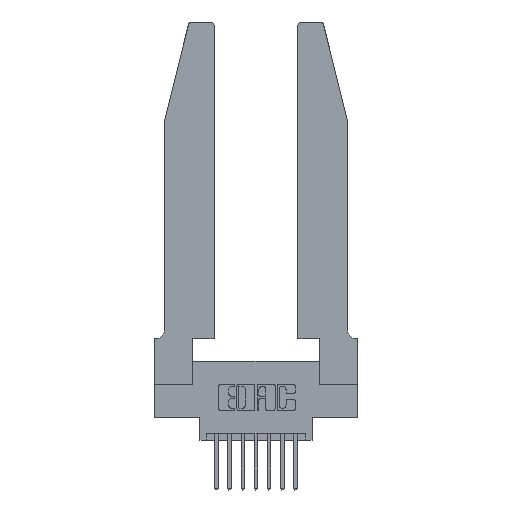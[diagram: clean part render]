
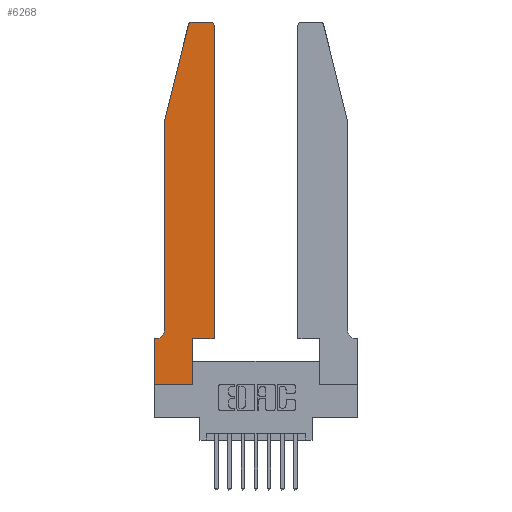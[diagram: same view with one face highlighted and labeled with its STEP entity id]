
A CAD part, top view. The second image highlights one B-rep face of the part: STEP entity #6268.
In plain terms, the highlighted planar face has unit normal (0, 0, 1).
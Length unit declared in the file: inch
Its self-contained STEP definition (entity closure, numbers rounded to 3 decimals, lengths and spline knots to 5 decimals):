
#168 = PLANE ( 'NONE',  #6182 ) ;
#201 = LINE ( 'NONE', #10219, #4741 ) ;
#325 = CARTESIAN_POINT ( 'NONE',  ( 0.2605, 2.75, 0.37 ) ) ;
#333 = CARTESIAN_POINT ( 'NONE',  ( 0.25487, 2.72718, 0.37 ) ) ;
#582 = EDGE_CURVE ( 'NONE', #6968, #1388, #7446, .T. ) ;
#644 = AXIS2_PLACEMENT_3D ( 'NONE', #13513, #14872, #884 ) ;
#813 = AXIS2_PLACEMENT_3D ( 'NONE', #11903, #7226, #1496 ) ;
#844 = ORIENTED_EDGE ( 'NONE', *, *, #5226, .T. ) ;
#884 = DIRECTION ( 'NONE',  ( 1., 0., 0. ) ) ;
#895 = LINE ( 'NONE', #1168, #10891 ) ;
#1052 = CIRCLE ( 'NONE', #7190, 0.03 ) ;
#1168 = CARTESIAN_POINT ( 'NONE',  ( 0.0755, 0.35, 0.37 ) ) ;
#1303 = ORIENTED_EDGE ( 'NONE', *, *, #3706, .T. ) ;
#1388 = VERTEX_POINT ( 'NONE', #13050 ) ;
#1453 = LINE ( 'NONE', #325, #6697 ) ;
#1496 = DIRECTION ( 'NONE',  ( -1., 0., 0. ) ) ;
#1751 = ORIENTED_EDGE ( 'NONE', *, *, #6201, .T. ) ;
#1813 = CARTESIAN_POINT ( 'NONE',  ( 0.2865, 0.35, 0.37 ) ) ;
#1966 = VECTOR ( 'NONE', #7671, 39.37008 ) ;
#2063 = EDGE_CURVE ( 'NONE', #12462, #11241, #1453, .T. ) ;
#2117 = ORIENTED_EDGE ( 'NONE', *, *, #2491, .T. ) ;
#2491 = EDGE_CURVE ( 'NONE', #1388, #6973, #895, .T. ) ;
#2629 = DIRECTION ( 'NONE',  ( 0., -1., 0. ) ) ;
#2671 = LINE ( 'NONE', #13246, #11955 ) ;
#2786 = CARTESIAN_POINT ( 'NONE',  ( 0., 0., 0.37 ) ) ;
#2813 = DIRECTION ( 'NONE',  ( 1., 0., 0. ) ) ;
#2815 = CARTESIAN_POINT ( 'NONE',  ( 0., 0., 0.37 ) ) ;
#3256 = CARTESIAN_POINT ( 'NONE',  ( 0.2865, 0., 0.37 ) ) ;
#3304 = DIRECTION ( 'NONE',  ( 0., 1., 0. ) ) ;
#3486 = CARTESIAN_POINT ( 'NONE',  ( 0.0755, 2., 0.37 ) ) ;
#3706 = EDGE_CURVE ( 'NONE', #4061, #13026, #6099, .T. ) ;
#3742 = LINE ( 'NONE', #2786, #11026 ) ;
#3994 = DIRECTION ( 'NONE',  ( -1., 0., 0. ) ) ;
#4061 = VERTEX_POINT ( 'NONE', #3256 ) ;
#4136 = DIRECTION ( 'NONE',  ( 0., 1., 0. ) ) ;
#4289 = EDGE_CURVE ( 'NONE', #11241, #5886, #12460, .T. ) ;
#4650 = DIRECTION ( 'NONE',  ( 1., 0., 0. ) ) ;
#4741 = VECTOR ( 'NONE', #3304, 39.37008 ) ;
#4876 = VECTOR ( 'NONE', #2813, 39.37008 ) ;
#5100 = DIRECTION ( 'NONE',  ( 0., -1., 0. ) ) ;
#5226 = EDGE_CURVE ( 'NONE', #5441, #14145, #201, .T. ) ;
#5325 = ORIENTED_EDGE ( 'NONE', *, *, #582, .T. ) ;
#5353 = CARTESIAN_POINT ( 'NONE',  ( 0., 0., 0.37 ) ) ;
#5441 = VERTEX_POINT ( 'NONE', #13183 ) ;
#5478 = CARTESIAN_POINT ( 'NONE',  ( 0.0755, 2., 0.37 ) ) ;
#5739 = VECTOR ( 'NONE', #4136, 39.37008 ) ;
#5886 = VERTEX_POINT ( 'NONE', #333 ) ;
#6099 = LINE ( 'NONE', #1813, #5739 ) ;
#6182 = AXIS2_PLACEMENT_3D ( 'NONE', #6960, #9442, #4650 ) ;
#6201 = EDGE_CURVE ( 'NONE', #5886, #10169, #8718, .T. ) ;
#6268 = ADVANCED_FACE ( 'NONE', ( #7607 ), #168, .T. ) ;
#6555 = EDGE_CURVE ( 'NONE', #13026, #5441, #13861, .T. ) ;
#6580 = ORIENTED_EDGE ( 'NONE', *, *, #2063, .T. ) ;
#6697 = VECTOR ( 'NONE', #3994, 39.37008 ) ;
#6746 = CARTESIAN_POINT ( 'NONE',  ( 0.284, 2.75, 0.37 ) ) ;
#6960 = CARTESIAN_POINT ( 'NONE',  ( 0., 0.35, 0.37 ) ) ;
#6968 = VERTEX_POINT ( 'NONE', #9806 ) ;
#6973 = VERTEX_POINT ( 'NONE', #7425 ) ;
#7037 = CARTESIAN_POINT ( 'NONE',  ( 0.2865, 0.35, 0.37 ) ) ;
#7072 = VECTOR ( 'NONE', #7097, 39.37008 ) ;
#7097 = DIRECTION ( 'NONE',  ( -0.239, -0.971, 0. ) ) ;
#7190 = AXIS2_PLACEMENT_3D ( 'NONE', #13823, #9083, #12634 ) ;
#7226 = DIRECTION ( 'NONE',  ( 0., 0., -1. ) ) ;
#7288 = ORIENTED_EDGE ( 'NONE', *, *, #4289, .T. ) ;
#7425 = CARTESIAN_POINT ( 'NONE',  ( 0., 0.35, 0.37 ) ) ;
#7446 = CIRCLE ( 'NONE', #813, 0.07 ) ;
#7607 = FACE_OUTER_BOUND ( 'NONE', #12505, .T. ) ;
#7671 = DIRECTION ( 'NONE',  ( 1., 0., 0. ) ) ;
#8292 = EDGE_CURVE ( 'NONE', #10169, #6968, #2671, .T. ) ;
#8718 = LINE ( 'NONE', #3486, #7072 ) ;
#9083 = DIRECTION ( 'NONE',  ( 0., 0., 1. ) ) ;
#9200 = LINE ( 'NONE', #5353, #1966 ) ;
#9302 = DIRECTION ( 'NONE',  ( -1., 0., 0. ) ) ;
#9442 = DIRECTION ( 'NONE',  ( 0., 0., 1. ) ) ;
#9769 = CARTESIAN_POINT ( 'NONE',  ( 0.4505, 0.35, 0.37 ) ) ;
#9806 = CARTESIAN_POINT ( 'NONE',  ( 0.0755, 0.42, 0.37 ) ) ;
#10169 = VERTEX_POINT ( 'NONE', #5478 ) ;
#10219 = CARTESIAN_POINT ( 'NONE',  ( 0.4505, 0.35, 0.37 ) ) ;
#10345 = ORIENTED_EDGE ( 'NONE', *, *, #8292, .T. ) ;
#10571 = ORIENTED_EDGE ( 'NONE', *, *, #11983, .T. ) ;
#10890 = ORIENTED_EDGE ( 'NONE', *, *, #12123, .T. ) ;
#10891 = VECTOR ( 'NONE', #9302, 39.37008 ) ;
#10973 = ORIENTED_EDGE ( 'NONE', *, *, #6555, .T. ) ;
#11026 = VECTOR ( 'NONE', #2629, 39.37008 ) ;
#11241 = VERTEX_POINT ( 'NONE', #6746 ) ;
#11269 = ORIENTED_EDGE ( 'NONE', *, *, #11650, .T. ) ;
#11650 = EDGE_CURVE ( 'NONE', #14145, #12462, #1052, .T. ) ;
#11903 = CARTESIAN_POINT ( 'NONE',  ( 0.0055, 0.42, 0.37 ) ) ;
#11955 = VECTOR ( 'NONE', #5100, 39.37008 ) ;
#11983 = EDGE_CURVE ( 'NONE', #6973, #13923, #3742, .T. ) ;
#12123 = EDGE_CURVE ( 'NONE', #13923, #4061, #9200, .T. ) ;
#12439 = CARTESIAN_POINT ( 'NONE',  ( 0.4505, 2.72, 0.37 ) ) ;
#12460 = CIRCLE ( 'NONE', #644, 0.03 ) ;
#12462 = VERTEX_POINT ( 'NONE', #12909 ) ;
#12505 = EDGE_LOOP ( 'NONE', ( #6580, #7288, #1751, #10345, #5325, #2117, #10571, #10890, #1303, #10973, #844, #11269 ) ) ;
#12634 = DIRECTION ( 'NONE',  ( 1., 0., 0. ) ) ;
#12909 = CARTESIAN_POINT ( 'NONE',  ( 0.4205, 2.75, 0.37 ) ) ;
#13026 = VERTEX_POINT ( 'NONE', #7037 ) ;
#13050 = CARTESIAN_POINT ( 'NONE',  ( 0.0055, 0.35, 0.37 ) ) ;
#13183 = CARTESIAN_POINT ( 'NONE',  ( 0.4505, 0.35, 0.37 ) ) ;
#13246 = CARTESIAN_POINT ( 'NONE',  ( 0.0755, 2., 0.37 ) ) ;
#13513 = CARTESIAN_POINT ( 'NONE',  ( 0.284, 2.72, 0.37 ) ) ;
#13823 = CARTESIAN_POINT ( 'NONE',  ( 0.4205, 2.72, 0.37 ) ) ;
#13861 = LINE ( 'NONE', #9769, #4876 ) ;
#13923 = VERTEX_POINT ( 'NONE', #2815 ) ;
#14145 = VERTEX_POINT ( 'NONE', #12439 ) ;
#14872 = DIRECTION ( 'NONE',  ( 0., 0., 1. ) ) ;
